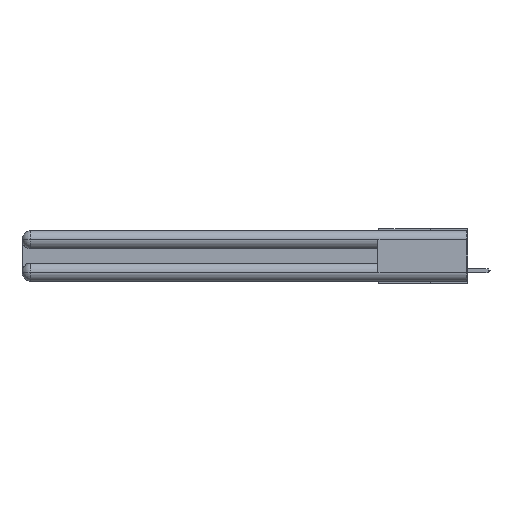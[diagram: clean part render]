
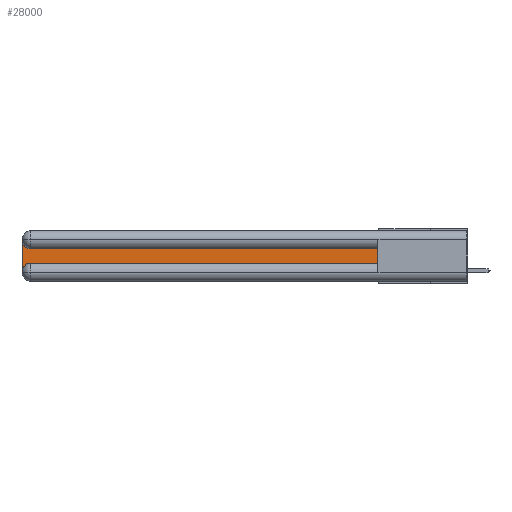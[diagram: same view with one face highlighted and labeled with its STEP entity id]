
A CAD part, left-side view. The second image highlights one B-rep face of the part: STEP entity #28000.
In plain terms, the highlighted planar face has unit normal (-1, 0, 0).
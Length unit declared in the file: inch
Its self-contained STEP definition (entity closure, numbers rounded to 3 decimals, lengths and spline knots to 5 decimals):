
#400 = DIRECTION ( 'NONE',  ( 0., 0., -1. ) ) ;
#660 = VERTEX_POINT ( 'NONE', #19952 ) ;
#704 = ORIENTED_EDGE ( 'NONE', *, *, #26714, .T. ) ;
#934 = CARTESIAN_POINT ( 'NONE',  ( 0.075, 3., -0.0625 ) ) ;
#1158 = CARTESIAN_POINT ( 'NONE',  ( 0.075, 2.94, -0.1225 ) ) ;
#1180 = CARTESIAN_POINT ( 'NONE',  ( 0.075, 3., -0.1225 ) ) ;
#2299 = DIRECTION ( 'NONE',  ( 0., 0., 1. ) ) ;
#2336 = EDGE_LOOP ( 'NONE', ( #15007, #16917, #14779, #17186, #24582, #704 ) ) ;
#2632 = LINE ( 'NONE', #20118, #13940 ) ;
#3233 = DIRECTION ( 'NONE',  ( 0., 0., -1. ) ) ;
#4284 = LINE ( 'NONE', #27478, #12523 ) ;
#4348 = DIRECTION ( 'NONE',  ( 0., -1., 0. ) ) ;
#4808 = CARTESIAN_POINT ( 'NONE',  ( 0.075, 2.94, -0.2775 ) ) ;
#4878 = VERTEX_POINT ( 'NONE', #26618 ) ;
#5870 = DIRECTION ( 'NONE',  ( 0., 0., -1. ) ) ;
#6160 = EDGE_CURVE ( 'NONE', #4878, #9730, #4284, .T. ) ;
#8225 = VERTEX_POINT ( 'NONE', #9420 ) ;
#8385 = VERTEX_POINT ( 'NONE', #934 ) ;
#9420 = CARTESIAN_POINT ( 'NONE',  ( 0.075, 2.94, -0.2175 ) ) ;
#9730 = VERTEX_POINT ( 'NONE', #1158 ) ;
#10022 = CIRCLE ( 'NONE', #11360, 0.06 ) ;
#11079 = VECTOR ( 'NONE', #14963, 39.37008 ) ;
#11360 = AXIS2_PLACEMENT_3D ( 'NONE', #16312, #27383, #3233 ) ;
#12379 = PLANE ( 'NONE',  #20675 ) ;
#12523 = VECTOR ( 'NONE', #16409, 39.37008 ) ;
#12686 = CARTESIAN_POINT ( 'NONE',  ( 0.075, 3., -0.2175 ) ) ;
#13137 = VECTOR ( 'NONE', #4348, 39.37008 ) ;
#13940 = VECTOR ( 'NONE', #2299, 39.37008 ) ;
#14779 = ORIENTED_EDGE ( 'NONE', *, *, #21435, .T. ) ;
#14794 = EDGE_CURVE ( 'NONE', #8225, #17854, #26090, .T. ) ;
#14963 = DIRECTION ( 'NONE',  ( 0., 0., -1. ) ) ;
#15007 = ORIENTED_EDGE ( 'NONE', *, *, #6160, .T. ) ;
#15582 = EDGE_CURVE ( 'NONE', #9730, #8385, #10022, .T. ) ;
#16312 = CARTESIAN_POINT ( 'NONE',  ( 0.075, 2.94, -0.0625 ) ) ;
#16409 = DIRECTION ( 'NONE',  ( 0., 1., 0. ) ) ;
#16917 = ORIENTED_EDGE ( 'NONE', *, *, #15582, .T. ) ;
#17186 = ORIENTED_EDGE ( 'NONE', *, *, #26854, .T. ) ;
#17854 = VERTEX_POINT ( 'NONE', #17963 ) ;
#17963 = CARTESIAN_POINT ( 'NONE',  ( 0.075, 0.6, -0.2175 ) ) ;
#19259 = FACE_OUTER_BOUND ( 'NONE', #2336, .T. ) ;
#19918 = LINE ( 'NONE', #12686, #11079 ) ;
#19952 = CARTESIAN_POINT ( 'NONE',  ( 0.075, 3., -0.2775 ) ) ;
#20118 = CARTESIAN_POINT ( 'NONE',  ( 0.075, 0.6, -0.2175 ) ) ;
#20165 = DIRECTION ( 'NONE',  ( 1., 0., 0. ) ) ;
#20675 = AXIS2_PLACEMENT_3D ( 'NONE', #1180, #23112, #5870 ) ;
#21435 = EDGE_CURVE ( 'NONE', #8385, #660, #19918, .T. ) ;
#23112 = DIRECTION ( 'NONE',  ( 1., 0., 0. ) ) ;
#24582 = ORIENTED_EDGE ( 'NONE', *, *, #14794, .T. ) ;
#25499 = CIRCLE ( 'NONE', #26740, 0.06 ) ;
#26090 = LINE ( 'NONE', #28069, #13137 ) ;
#26618 = CARTESIAN_POINT ( 'NONE',  ( 0.075, 0.6, -0.1225 ) ) ;
#26714 = EDGE_CURVE ( 'NONE', #17854, #4878, #2632, .T. ) ;
#26740 = AXIS2_PLACEMENT_3D ( 'NONE', #4808, #20165, #400 ) ;
#26854 = EDGE_CURVE ( 'NONE', #660, #8225, #25499, .T. ) ;
#27383 = DIRECTION ( 'NONE',  ( 1., 0., 0. ) ) ;
#27478 = CARTESIAN_POINT ( 'NONE',  ( 0.075, 0.6, -0.1225 ) ) ;
#28000 = ADVANCED_FACE ( 'NONE', ( #19259 ), #12379, .F. ) ;
#28069 = CARTESIAN_POINT ( 'NONE',  ( 0.075, 0.6, -0.2175 ) ) ;
